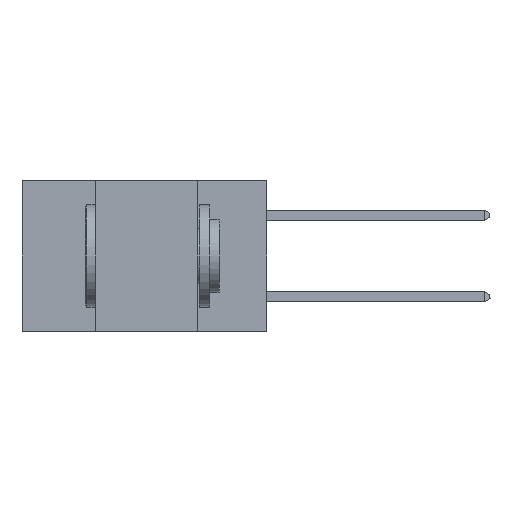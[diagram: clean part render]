
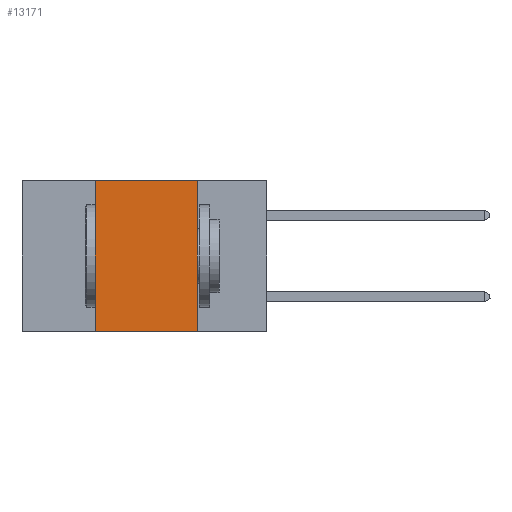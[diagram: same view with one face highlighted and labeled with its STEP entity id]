
A CAD part, left-side view. The second image highlights one B-rep face of the part: STEP entity #13171.
In plain terms, the highlighted planar face has unit normal (-1, 0, 0).
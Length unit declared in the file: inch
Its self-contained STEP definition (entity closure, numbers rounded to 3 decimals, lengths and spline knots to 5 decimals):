
#90 = VECTOR ( 'NONE', #10275, 39.37008 ) ;
#416 = CARTESIAN_POINT ( 'NONE',  ( 0., 0.6, 0. ) ) ;
#1168 = CARTESIAN_POINT ( 'NONE',  ( 0., 0.42, 0. ) ) ;
#1302 = ORIENTED_EDGE ( 'NONE', *, *, #9177, .F. ) ;
#2168 = LINE ( 'NONE', #1168, #15861 ) ;
#2570 = EDGE_CURVE ( 'NONE', #5356, #15054, #7779, .T. ) ;
#2632 = CARTESIAN_POINT ( 'NONE',  ( 0., 0.42, 0. ) ) ;
#3596 = PLANE ( 'NONE',  #20728 ) ;
#5356 = VERTEX_POINT ( 'NONE', #9137 ) ;
#5592 = ORIENTED_EDGE ( 'NONE', *, *, #17795, .F. ) ;
#6064 = LINE ( 'NONE', #10135, #90 ) ;
#6708 = ORIENTED_EDGE ( 'NONE', *, *, #21356, .F. ) ;
#6725 = CARTESIAN_POINT ( 'NONE',  ( 0., 0.17, 0. ) ) ;
#7003 = VECTOR ( 'NONE', #11079, 39.37008 ) ;
#7762 = CARTESIAN_POINT ( 'NONE',  ( 0., 0.6, -0.37 ) ) ;
#7779 = LINE ( 'NONE', #7762, #7003 ) ;
#9137 = CARTESIAN_POINT ( 'NONE',  ( 0., 0.42, -0.37 ) ) ;
#9177 = EDGE_CURVE ( 'NONE', #18578, #15054, #6064, .T. ) ;
#10135 = CARTESIAN_POINT ( 'NONE',  ( 0., 0.17, 0. ) ) ;
#10275 = DIRECTION ( 'NONE',  ( 0., 0., -1. ) ) ;
#10576 = FACE_OUTER_BOUND ( 'NONE', #14492, .T. ) ;
#11079 = DIRECTION ( 'NONE',  ( 0., -1., 0. ) ) ;
#11104 = DIRECTION ( 'NONE',  ( 0., -1., 0. ) ) ;
#13171 = ADVANCED_FACE ( 'NONE', ( #10576 ), #3596, .F. ) ;
#13507 = DIRECTION ( 'NONE',  ( 0., 0., -1. ) ) ;
#14260 = CARTESIAN_POINT ( 'NONE',  ( 0., 0.6, 0. ) ) ;
#14492 = EDGE_LOOP ( 'NONE', ( #1302, #6708, #5592, #15603 ) ) ;
#14948 = VECTOR ( 'NONE', #11104, 39.37008 ) ;
#15054 = VERTEX_POINT ( 'NONE', #18767 ) ;
#15603 = ORIENTED_EDGE ( 'NONE', *, *, #2570, .T. ) ;
#15757 = DIRECTION ( 'NONE',  ( 0., 0., 1. ) ) ;
#15861 = VECTOR ( 'NONE', #15757, 39.37008 ) ;
#17795 = EDGE_CURVE ( 'NONE', #5356, #17858, #2168, .T. ) ;
#17858 = VERTEX_POINT ( 'NONE', #2632 ) ;
#18578 = VERTEX_POINT ( 'NONE', #6725 ) ;
#18767 = CARTESIAN_POINT ( 'NONE',  ( 0., 0.17, -0.37 ) ) ;
#19897 = LINE ( 'NONE', #14260, #14948 ) ;
#20092 = DIRECTION ( 'NONE',  ( 1., 0., 0. ) ) ;
#20728 = AXIS2_PLACEMENT_3D ( 'NONE', #416, #20092, #13507 ) ;
#21356 = EDGE_CURVE ( 'NONE', #17858, #18578, #19897, .T. ) ;
